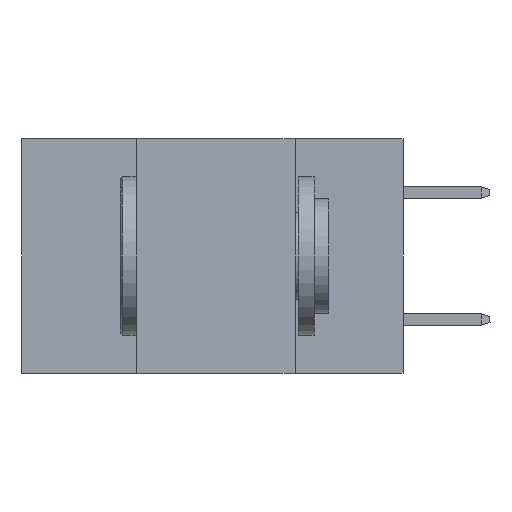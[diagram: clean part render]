
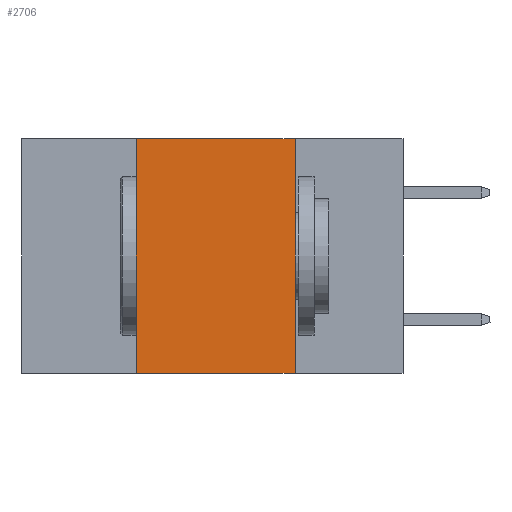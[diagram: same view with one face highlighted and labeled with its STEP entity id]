
A CAD part, left-side view. The second image highlights one B-rep face of the part: STEP entity #2706.
In plain terms, the highlighted planar face has unit normal (-1, 0, 0).
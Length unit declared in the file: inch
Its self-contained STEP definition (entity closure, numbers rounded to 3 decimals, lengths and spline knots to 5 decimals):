
#884 = AXIS2_PLACEMENT_3D ( 'NONE', #1640, #6423, #1727 ) ;
#1140 = DIRECTION ( 'NONE',  ( 0., 0., -1. ) ) ;
#1144 = DIRECTION ( 'NONE',  ( 0., 0., 1. ) ) ;
#1446 = CARTESIAN_POINT ( 'NONE',  ( 0., 0.42, 0. ) ) ;
#1626 = LINE ( 'NONE', #1786, #12017 ) ;
#1640 = CARTESIAN_POINT ( 'NONE',  ( 0., 0.6, 0. ) ) ;
#1656 = EDGE_CURVE ( 'NONE', #12200, #14423, #14272, .T. ) ;
#1727 = DIRECTION ( 'NONE',  ( 0., 0., -1. ) ) ;
#1786 = CARTESIAN_POINT ( 'NONE',  ( 0., 0.6, -0.37 ) ) ;
#2058 = DIRECTION ( 'NONE',  ( 0., -1., 0. ) ) ;
#2706 = ADVANCED_FACE ( 'NONE', ( #14857 ), #2909, .F. ) ;
#2909 = PLANE ( 'NONE',  #884 ) ;
#3154 = CARTESIAN_POINT ( 'NONE',  ( 0., 0.17, 0. ) ) ;
#4793 = ORIENTED_EDGE ( 'NONE', *, *, #8090, .T. ) ;
#5165 = VERTEX_POINT ( 'NONE', #9838 ) ;
#5247 = VECTOR ( 'NONE', #2058, 39.37008 ) ;
#5786 = LINE ( 'NONE', #14266, #11619 ) ;
#5930 = VERTEX_POINT ( 'NONE', #3154 ) ;
#6061 = ORIENTED_EDGE ( 'NONE', *, *, #12074, .F. ) ;
#6392 = ORIENTED_EDGE ( 'NONE', *, *, #7413, .F. ) ;
#6423 = DIRECTION ( 'NONE',  ( 1., 0., 0. ) ) ;
#7413 = EDGE_CURVE ( 'NONE', #14423, #5930, #9366, .T. ) ;
#8090 = EDGE_CURVE ( 'NONE', #12200, #5165, #1626, .T. ) ;
#9366 = LINE ( 'NONE', #15197, #5247 ) ;
#9545 = VECTOR ( 'NONE', #1144, 39.37008 ) ;
#9838 = CARTESIAN_POINT ( 'NONE',  ( 0., 0.17, -0.37 ) ) ;
#10394 = CARTESIAN_POINT ( 'NONE',  ( 0., 0.42, -0.37 ) ) ;
#11220 = DIRECTION ( 'NONE',  ( 0., -1., 0. ) ) ;
#11619 = VECTOR ( 'NONE', #1140, 39.37008 ) ;
#11943 = CARTESIAN_POINT ( 'NONE',  ( 0., 0.42, 0. ) ) ;
#12017 = VECTOR ( 'NONE', #11220, 39.37008 ) ;
#12025 = ORIENTED_EDGE ( 'NONE', *, *, #1656, .F. ) ;
#12074 = EDGE_CURVE ( 'NONE', #5930, #5165, #5786, .T. ) ;
#12200 = VERTEX_POINT ( 'NONE', #10394 ) ;
#13121 = EDGE_LOOP ( 'NONE', ( #6061, #6392, #12025, #4793 ) ) ;
#14266 = CARTESIAN_POINT ( 'NONE',  ( 0., 0.17, 0. ) ) ;
#14272 = LINE ( 'NONE', #11943, #9545 ) ;
#14423 = VERTEX_POINT ( 'NONE', #1446 ) ;
#14857 = FACE_OUTER_BOUND ( 'NONE', #13121, .T. ) ;
#15197 = CARTESIAN_POINT ( 'NONE',  ( 0., 0.6, 0. ) ) ;
